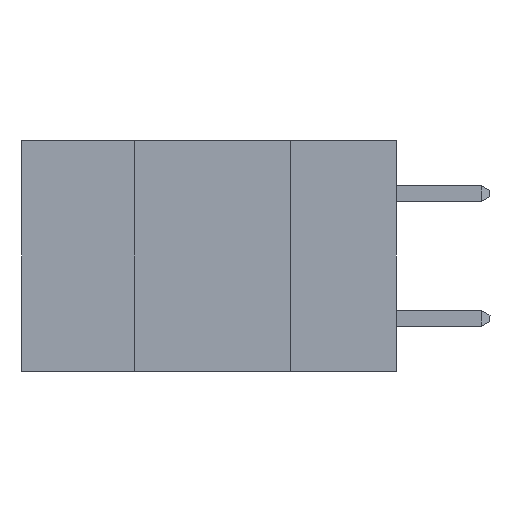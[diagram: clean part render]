
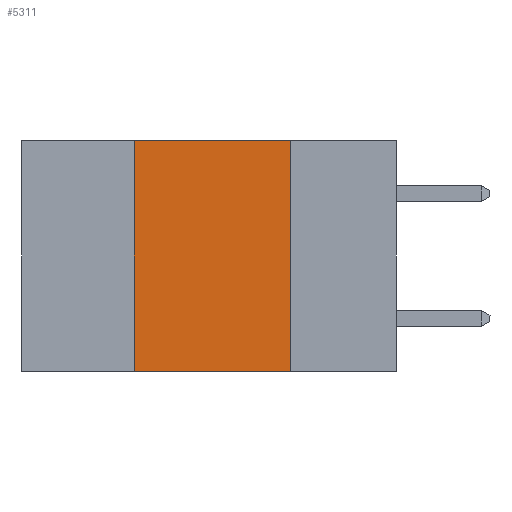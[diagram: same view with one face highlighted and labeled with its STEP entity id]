
A CAD part, left-side view. The second image highlights one B-rep face of the part: STEP entity #5311.
In plain terms, the highlighted planar face has unit normal (-1, 0, 0).
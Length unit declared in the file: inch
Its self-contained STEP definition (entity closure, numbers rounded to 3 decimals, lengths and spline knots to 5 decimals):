
#210 = AXIS2_PLACEMENT_3D ( 'NONE', #5491, #4484, #4414 ) ;
#412 = VECTOR ( 'NONE', #1933, 39.37008 ) ;
#511 = VERTEX_POINT ( 'NONE', #2712 ) ;
#840 = EDGE_CURVE ( 'NONE', #3755, #6578, #7659, .T. ) ;
#1300 = VECTOR ( 'NONE', #2924, 39.37008 ) ;
#1523 = CARTESIAN_POINT ( 'NONE',  ( 0., 0.17, -0.37 ) ) ;
#1758 = CARTESIAN_POINT ( 'NONE',  ( 0., 0.42, -0.37 ) ) ;
#1778 = DIRECTION ( 'NONE',  ( 0., 0., 1. ) ) ;
#1933 = DIRECTION ( 'NONE',  ( 0., -1., 0. ) ) ;
#2512 = CARTESIAN_POINT ( 'NONE',  ( 0., 0.6, -0.37 ) ) ;
#2577 = VECTOR ( 'NONE', #1778, 39.37008 ) ;
#2712 = CARTESIAN_POINT ( 'NONE',  ( 0., 0.17, 0. ) ) ;
#2777 = LINE ( 'NONE', #1758, #2577 ) ;
#2924 = DIRECTION ( 'NONE',  ( 0., 0., -1. ) ) ;
#3151 = LINE ( 'NONE', #3517, #1300 ) ;
#3333 = VECTOR ( 'NONE', #6907, 39.37008 ) ;
#3517 = CARTESIAN_POINT ( 'NONE',  ( 0., 0.17, -0.37 ) ) ;
#3755 = VERTEX_POINT ( 'NONE', #3937 ) ;
#3937 = CARTESIAN_POINT ( 'NONE',  ( 0., 0.42, -0.37 ) ) ;
#4414 = DIRECTION ( 'NONE',  ( 0., 0., -1. ) ) ;
#4484 = DIRECTION ( 'NONE',  ( 1., 0., 0. ) ) ;
#4742 = LINE ( 'NONE', #6283, #3333 ) ;
#4995 = VERTEX_POINT ( 'NONE', #6948 ) ;
#5296 = EDGE_CURVE ( 'NONE', #4995, #511, #4742, .T. ) ;
#5311 = ADVANCED_FACE ( 'NONE', ( #7781 ), #5424, .F. ) ;
#5424 = PLANE ( 'NONE',  #210 ) ;
#5491 = CARTESIAN_POINT ( 'NONE',  ( 0., 0.6, 0. ) ) ;
#5860 = EDGE_LOOP ( 'NONE', ( #8001, #6275, #6295, #6320 ) ) ;
#6275 = ORIENTED_EDGE ( 'NONE', *, *, #5296, .F. ) ;
#6283 = CARTESIAN_POINT ( 'NONE',  ( 0., 0.6, 0. ) ) ;
#6295 = ORIENTED_EDGE ( 'NONE', *, *, #6568, .F. ) ;
#6320 = ORIENTED_EDGE ( 'NONE', *, *, #840, .T. ) ;
#6568 = EDGE_CURVE ( 'NONE', #3755, #4995, #2777, .T. ) ;
#6578 = VERTEX_POINT ( 'NONE', #1523 ) ;
#6907 = DIRECTION ( 'NONE',  ( 0., -1., 0. ) ) ;
#6948 = CARTESIAN_POINT ( 'NONE',  ( 0., 0.42, 0. ) ) ;
#7534 = EDGE_CURVE ( 'NONE', #511, #6578, #3151, .T. ) ;
#7659 = LINE ( 'NONE', #2512, #412 ) ;
#7781 = FACE_OUTER_BOUND ( 'NONE', #5860, .T. ) ;
#8001 = ORIENTED_EDGE ( 'NONE', *, *, #7534, .F. ) ;
